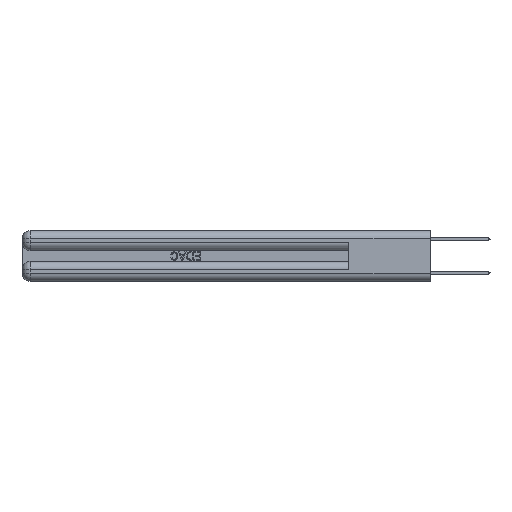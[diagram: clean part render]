
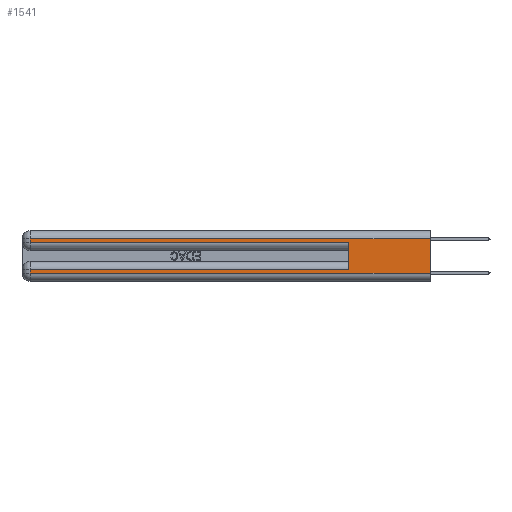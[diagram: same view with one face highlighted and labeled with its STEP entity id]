
A CAD part, left-side view. The second image highlights one B-rep face of the part: STEP entity #1541.
In plain terms, the highlighted planar face has unit normal (-1, 0, 0).
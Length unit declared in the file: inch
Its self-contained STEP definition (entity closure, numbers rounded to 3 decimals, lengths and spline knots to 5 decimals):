
#541 = VECTOR ( 'NONE', #30024, 39.37008 ) ;
#783 = VECTOR ( 'NONE', #28929, 39.37008 ) ;
#824 = ORIENTED_EDGE ( 'NONE', *, *, #8486, .T. ) ;
#1541 = ADVANCED_FACE ( 'NONE', ( #9597 ), #15347, .F. ) ;
#2220 = EDGE_CURVE ( 'NONE', #2978, #13120, #19490, .T. ) ;
#2407 = CARTESIAN_POINT ( 'NONE',  ( 0., 0., 0.285 ) ) ;
#2605 = EDGE_CURVE ( 'NONE', #16286, #20122, #31347, .T. ) ;
#2651 = VECTOR ( 'NONE', #16400, 39.37008 ) ;
#2978 = VERTEX_POINT ( 'NONE', #16358 ) ;
#3372 = DIRECTION ( 'NONE',  ( 0., 0., -1. ) ) ;
#4203 = VECTOR ( 'NONE', #16849, 39.37008 ) ;
#4794 = VERTEX_POINT ( 'NONE', #9621 ) ;
#5208 = ORIENTED_EDGE ( 'NONE', *, *, #9119, .T. ) ;
#5363 = CARTESIAN_POINT ( 'NONE',  ( 0., 2.94, 0.06 ) ) ;
#5483 = CARTESIAN_POINT ( 'NONE',  ( 0., 2.94, 0.37 ) ) ;
#6073 = CARTESIAN_POINT ( 'NONE',  ( 0., 0., 0.37 ) ) ;
#6889 = EDGE_CURVE ( 'NONE', #2978, #16326, #26869, .T. ) ;
#7058 = DIRECTION ( 'NONE',  ( 0., 0., -1. ) ) ;
#7757 = VERTEX_POINT ( 'NONE', #27461 ) ;
#8129 = ORIENTED_EDGE ( 'NONE', *, *, #2605, .F. ) ;
#8486 = EDGE_CURVE ( 'NONE', #14516, #20122, #20300, .T. ) ;
#8858 = EDGE_LOOP ( 'NONE', ( #8129, #28806, #18833, #25687, #22740, #13726, #5208, #824 ) ) ;
#9030 = CARTESIAN_POINT ( 'NONE',  ( 0., 0.6, 0.145 ) ) ;
#9119 = EDGE_CURVE ( 'NONE', #13120, #14516, #18367, .T. ) ;
#9226 = CARTESIAN_POINT ( 'NONE',  ( 0., 0., 0.06 ) ) ;
#9597 = FACE_OUTER_BOUND ( 'NONE', #8858, .T. ) ;
#9621 = CARTESIAN_POINT ( 'NONE',  ( 0., 2.94, 0.31 ) ) ;
#10311 = EDGE_CURVE ( 'NONE', #7757, #16326, #17705, .T. ) ;
#12794 = CARTESIAN_POINT ( 'NONE',  ( 0., 0., 0.31 ) ) ;
#13120 = VERTEX_POINT ( 'NONE', #24125 ) ;
#13726 = ORIENTED_EDGE ( 'NONE', *, *, #2220, .T. ) ;
#14516 = VERTEX_POINT ( 'NONE', #5363 ) ;
#15347 = PLANE ( 'NONE',  #24598 ) ;
#15594 = VECTOR ( 'NONE', #15823, 39.37008 ) ;
#15823 = DIRECTION ( 'NONE',  ( 0., 0., -1. ) ) ;
#16273 = CARTESIAN_POINT ( 'NONE',  ( 0., 2.94, 0.37 ) ) ;
#16286 = VERTEX_POINT ( 'NONE', #12794 ) ;
#16326 = VERTEX_POINT ( 'NONE', #17342 ) ;
#16358 = CARTESIAN_POINT ( 'NONE',  ( 0., 0.6, 0.085 ) ) ;
#16400 = DIRECTION ( 'NONE',  ( 0., 0., -1. ) ) ;
#16849 = DIRECTION ( 'NONE',  ( 0., 0., 1. ) ) ;
#17342 = CARTESIAN_POINT ( 'NONE',  ( 0., 0.6, 0.285 ) ) ;
#17705 = LINE ( 'NONE', #2407, #26497 ) ;
#18367 = LINE ( 'NONE', #5483, #15594 ) ;
#18833 = ORIENTED_EDGE ( 'NONE', *, *, #30097, .T. ) ;
#19490 = LINE ( 'NONE', #19662, #541 ) ;
#19662 = CARTESIAN_POINT ( 'NONE',  ( 0., 0., 0.085 ) ) ;
#19950 = CARTESIAN_POINT ( 'NONE',  ( 0., 0., 0.37 ) ) ;
#20122 = VERTEX_POINT ( 'NONE', #9226 ) ;
#20300 = LINE ( 'NONE', #28105, #24300 ) ;
#21533 = LINE ( 'NONE', #16273, #27081 ) ;
#22209 = EDGE_CURVE ( 'NONE', #16286, #4794, #31474, .T. ) ;
#22740 = ORIENTED_EDGE ( 'NONE', *, *, #6889, .F. ) ;
#23126 = DIRECTION ( 'NONE',  ( 0., -1., 0. ) ) ;
#24125 = CARTESIAN_POINT ( 'NONE',  ( 0., 2.94, 0.085 ) ) ;
#24300 = VECTOR ( 'NONE', #27939, 39.37008 ) ;
#24598 = AXIS2_PLACEMENT_3D ( 'NONE', #19950, #30313, #7058 ) ;
#25687 = ORIENTED_EDGE ( 'NONE', *, *, #10311, .T. ) ;
#26497 = VECTOR ( 'NONE', #23126, 39.37008 ) ;
#26869 = LINE ( 'NONE', #9030, #4203 ) ;
#27081 = VECTOR ( 'NONE', #3372, 39.37008 ) ;
#27461 = CARTESIAN_POINT ( 'NONE',  ( 0., 2.94, 0.285 ) ) ;
#27939 = DIRECTION ( 'NONE',  ( 0., -1., 0. ) ) ;
#28105 = CARTESIAN_POINT ( 'NONE',  ( 0., 0., 0.06 ) ) ;
#28806 = ORIENTED_EDGE ( 'NONE', *, *, #22209, .T. ) ;
#28929 = DIRECTION ( 'NONE',  ( 0., 1., 0. ) ) ;
#29089 = CARTESIAN_POINT ( 'NONE',  ( 0., 0., 0.31 ) ) ;
#30024 = DIRECTION ( 'NONE',  ( 0., 1., 0. ) ) ;
#30097 = EDGE_CURVE ( 'NONE', #4794, #7757, #21533, .T. ) ;
#30313 = DIRECTION ( 'NONE',  ( 1., 0., 0. ) ) ;
#31347 = LINE ( 'NONE', #6073, #2651 ) ;
#31474 = LINE ( 'NONE', #29089, #783 ) ;
